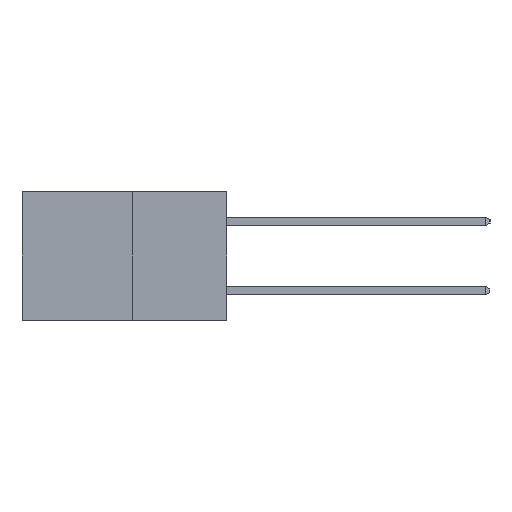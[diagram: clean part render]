
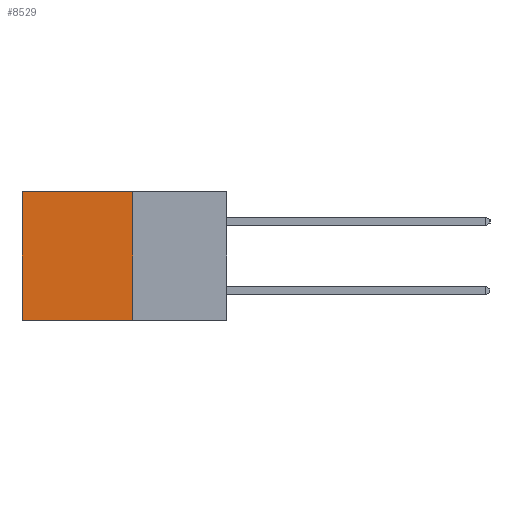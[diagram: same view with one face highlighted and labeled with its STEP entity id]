
A CAD part, left-side view. The second image highlights one B-rep face of the part: STEP entity #8529.
In plain terms, the highlighted planar face has unit normal (-1, 0, 0).
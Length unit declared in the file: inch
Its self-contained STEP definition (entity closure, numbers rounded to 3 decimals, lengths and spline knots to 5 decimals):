
#804 = DIRECTION ( 'NONE',  ( 0., 0., -1. ) ) ;
#1773 = EDGE_LOOP ( 'NONE', ( #12782, #12820, #14020, #14182 ) ) ;
#2074 = EDGE_CURVE ( 'NONE', #8658, #17137, #8610, .T. ) ;
#2323 = EDGE_CURVE ( 'NONE', #13680, #8658, #6991, .T. ) ;
#3109 = VERTEX_POINT ( 'NONE', #7430 ) ;
#3694 = PLANE ( 'NONE',  #15825 ) ;
#3894 = CARTESIAN_POINT ( 'NONE',  ( 0.277, 0.59, -0.37 ) ) ;
#4345 = FACE_OUTER_BOUND ( 'NONE', #1773, .T. ) ;
#5131 = CARTESIAN_POINT ( 'NONE',  ( 0.277, 0.27, -0.37 ) ) ;
#5805 = CARTESIAN_POINT ( 'NONE',  ( 0.277, 0.27, -0.37 ) ) ;
#6991 = LINE ( 'NONE', #7511, #10437 ) ;
#7244 = DIRECTION ( 'NONE',  ( 0., 1., 0. ) ) ;
#7419 = EDGE_CURVE ( 'NONE', #3109, #17137, #8081, .T. ) ;
#7430 = CARTESIAN_POINT ( 'NONE',  ( 0.277, 0.27, -0.37 ) ) ;
#7511 = CARTESIAN_POINT ( 'NONE',  ( 0.277, 0.27, 0. ) ) ;
#8081 = LINE ( 'NONE', #8776, #11513 ) ;
#8529 = ADVANCED_FACE ( 'NONE', ( #4345 ), #3694, .F. ) ;
#8610 = LINE ( 'NONE', #14409, #12048 ) ;
#8658 = VERTEX_POINT ( 'NONE', #10151 ) ;
#8776 = CARTESIAN_POINT ( 'NONE',  ( 0.277, 0.27, -0.37 ) ) ;
#9358 = EDGE_CURVE ( 'NONE', #13680, #3109, #13908, .T. ) ;
#9638 = DIRECTION ( 'NONE',  ( 1., 0., 0. ) ) ;
#10151 = CARTESIAN_POINT ( 'NONE',  ( 0.277, 0.59, 0. ) ) ;
#10437 = VECTOR ( 'NONE', #7244, 39.37008 ) ;
#11513 = VECTOR ( 'NONE', #18843, 39.37008 ) ;
#12048 = VECTOR ( 'NONE', #14691, 39.37008 ) ;
#12782 = ORIENTED_EDGE ( 'NONE', *, *, #2074, .T. ) ;
#12820 = ORIENTED_EDGE ( 'NONE', *, *, #7419, .F. ) ;
#13470 = VECTOR ( 'NONE', #18847, 39.37008 ) ;
#13680 = VERTEX_POINT ( 'NONE', #14534 ) ;
#13908 = LINE ( 'NONE', #5805, #13470 ) ;
#14020 = ORIENTED_EDGE ( 'NONE', *, *, #9358, .F. ) ;
#14182 = ORIENTED_EDGE ( 'NONE', *, *, #2323, .T. ) ;
#14409 = CARTESIAN_POINT ( 'NONE',  ( 0.277, 0.59, -0.37 ) ) ;
#14534 = CARTESIAN_POINT ( 'NONE',  ( 0.277, 0.27, 0. ) ) ;
#14691 = DIRECTION ( 'NONE',  ( 0., 0., -1. ) ) ;
#15825 = AXIS2_PLACEMENT_3D ( 'NONE', #5131, #9638, #804 ) ;
#17137 = VERTEX_POINT ( 'NONE', #3894 ) ;
#18843 = DIRECTION ( 'NONE',  ( 0., 1., 0. ) ) ;
#18847 = DIRECTION ( 'NONE',  ( 0., 0., -1. ) ) ;
